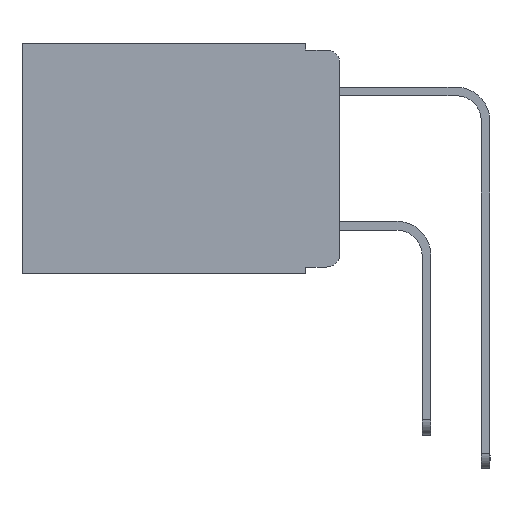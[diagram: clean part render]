
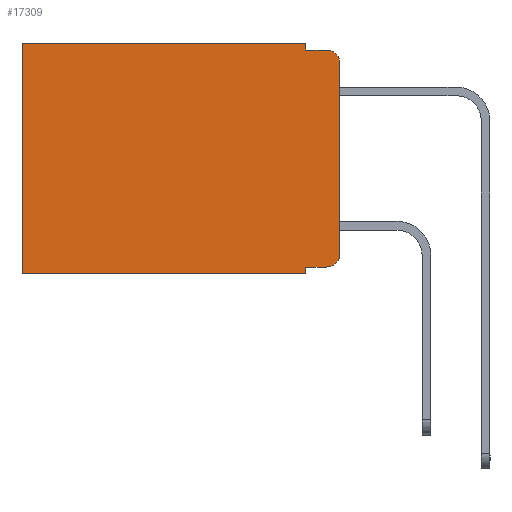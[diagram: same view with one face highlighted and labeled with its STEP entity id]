
A CAD part, left-side view. The second image highlights one B-rep face of the part: STEP entity #17309.
In plain terms, the highlighted planar face has unit normal (-1, 0, 0).
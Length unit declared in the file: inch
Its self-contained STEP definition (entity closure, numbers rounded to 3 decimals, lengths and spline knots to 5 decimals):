
#374 = VERTEX_POINT ( 'NONE', #19808 ) ;
#746 = AXIS2_PLACEMENT_3D ( 'NONE', #20291, #24024, #22146 ) ;
#793 = ORIENTED_EDGE ( 'NONE', *, *, #6416, .F. ) ;
#1081 = VERTEX_POINT ( 'NONE', #4981 ) ;
#1228 = CARTESIAN_POINT ( 'NONE',  ( 0.298, 0.473, -0.343 ) ) ;
#1316 = ORIENTED_EDGE ( 'NONE', *, *, #24752, .F. ) ;
#1496 = DIRECTION ( 'NONE',  ( 0., 0., -1. ) ) ;
#1647 = LINE ( 'NONE', #25582, #19690 ) ;
#1856 = CARTESIAN_POINT ( 'NONE',  ( 0.298, 0.051, -0.01 ) ) ;
#1897 = CARTESIAN_POINT ( 'NONE',  ( 0.298, 0., -0.313 ) ) ;
#3254 = DIRECTION ( 'NONE',  ( -1., 0., 0. ) ) ;
#3382 = DIRECTION ( 'NONE',  ( 0., 0., -1. ) ) ;
#3552 = LINE ( 'NONE', #17128, #19204 ) ;
#3572 = CARTESIAN_POINT ( 'NONE',  ( 0.298, 0., -0.343 ) ) ;
#3662 = FACE_OUTER_BOUND ( 'NONE', #3953, .T. ) ;
#3953 = EDGE_LOOP ( 'NONE', ( #14051, #13202, #793, #1316, #12378, #7994, #12371, #14739, #6467, #18732 ) ) ;
#4981 = CARTESIAN_POINT ( 'NONE',  ( 0.298, 0.051, 0. ) ) ;
#5083 = LINE ( 'NONE', #25435, #20933 ) ;
#5243 = VERTEX_POINT ( 'NONE', #13425 ) ;
#5363 = CIRCLE ( 'NONE', #21504, 0.02 ) ;
#6416 = EDGE_CURVE ( 'NONE', #20065, #8487, #1647, .T. ) ;
#6467 = ORIENTED_EDGE ( 'NONE', *, *, #23620, .T. ) ;
#6502 = EDGE_CURVE ( 'NONE', #1081, #5243, #12140, .T. ) ;
#6815 = VERTEX_POINT ( 'NONE', #1228 ) ;
#7169 = CARTESIAN_POINT ( 'NONE',  ( 0.298, 0.02, -0.01 ) ) ;
#7228 = DIRECTION ( 'NONE',  ( 0., -1., 0. ) ) ;
#7580 = EDGE_CURVE ( 'NONE', #374, #20787, #5363, .T. ) ;
#7651 = AXIS2_PLACEMENT_3D ( 'NONE', #17007, #13262, #10768 ) ;
#7803 = VECTOR ( 'NONE', #22971, 39.37008 ) ;
#7994 = ORIENTED_EDGE ( 'NONE', *, *, #25446, .T. ) ;
#8144 = EDGE_CURVE ( 'NONE', #11261, #20787, #21834, .T. ) ;
#8487 = VERTEX_POINT ( 'NONE', #7169 ) ;
#9439 = CARTESIAN_POINT ( 'NONE',  ( 0.298, 0.051, -0.343 ) ) ;
#9646 = CARTESIAN_POINT ( 'NONE',  ( 0.298, 0.02, -0.313 ) ) ;
#9894 = CARTESIAN_POINT ( 'NONE',  ( 0.298, 0., 0. ) ) ;
#9926 = VERTEX_POINT ( 'NONE', #9439 ) ;
#10768 = DIRECTION ( 'NONE',  ( 0., 0., -1. ) ) ;
#11077 = DIRECTION ( 'NONE',  ( 0., 0., -1. ) ) ;
#11261 = VERTEX_POINT ( 'NONE', #17435 ) ;
#12140 = LINE ( 'NONE', #9894, #23507 ) ;
#12351 = CARTESIAN_POINT ( 'NONE',  ( 0.298, 0.051, -0.333 ) ) ;
#12371 = ORIENTED_EDGE ( 'NONE', *, *, #14159, .F. ) ;
#12378 = ORIENTED_EDGE ( 'NONE', *, *, #6502, .T. ) ;
#12845 = CARTESIAN_POINT ( 'NONE',  ( 0.298, 0.473, 0. ) ) ;
#13202 = ORIENTED_EDGE ( 'NONE', *, *, #20263, .T. ) ;
#13262 = DIRECTION ( 'NONE',  ( -1., 0., 0. ) ) ;
#13425 = CARTESIAN_POINT ( 'NONE',  ( 0.298, 0.473, 0. ) ) ;
#13675 = DIRECTION ( 'NONE',  ( 0., 1., 0. ) ) ;
#14051 = ORIENTED_EDGE ( 'NONE', *, *, #8144, .F. ) ;
#14091 = DIRECTION ( 'NONE',  ( 0., -1., 0. ) ) ;
#14159 = EDGE_CURVE ( 'NONE', #9926, #6815, #21661, .T. ) ;
#14739 = ORIENTED_EDGE ( 'NONE', *, *, #23809, .F. ) ;
#15787 = VECTOR ( 'NONE', #14091, 39.37008 ) ;
#17007 = CARTESIAN_POINT ( 'NONE',  ( 0.298, 0.02, -0.03 ) ) ;
#17094 = LINE ( 'NONE', #12845, #7803 ) ;
#17128 = CARTESIAN_POINT ( 'NONE',  ( 0.298, 0.051, 0. ) ) ;
#17309 = ADVANCED_FACE ( 'NONE', ( #3662 ), #22421, .F. ) ;
#17435 = CARTESIAN_POINT ( 'NONE',  ( 0.298, 0., -0.03 ) ) ;
#18732 = ORIENTED_EDGE ( 'NONE', *, *, #7580, .T. ) ;
#19065 = CARTESIAN_POINT ( 'NONE',  ( 0.298, 0.051, -0.333 ) ) ;
#19204 = VECTOR ( 'NONE', #19257, 39.37008 ) ;
#19257 = DIRECTION ( 'NONE',  ( 0., 0., -1. ) ) ;
#19319 = VECTOR ( 'NONE', #1496, 39.37008 ) ;
#19453 = CARTESIAN_POINT ( 'NONE',  ( 0.298, 0., 0. ) ) ;
#19690 = VECTOR ( 'NONE', #7228, 39.37008 ) ;
#19808 = CARTESIAN_POINT ( 'NONE',  ( 0.298, 0.02, -0.333 ) ) ;
#20065 = VERTEX_POINT ( 'NONE', #1856 ) ;
#20078 = LINE ( 'NONE', #12351, #15787 ) ;
#20263 = EDGE_CURVE ( 'NONE', #11261, #8487, #20398, .T. ) ;
#20291 = CARTESIAN_POINT ( 'NONE',  ( 0.298, 0., 0. ) ) ;
#20398 = CIRCLE ( 'NONE', #7651, 0.02 ) ;
#20787 = VERTEX_POINT ( 'NONE', #1897 ) ;
#20933 = VECTOR ( 'NONE', #11077, 39.37008 ) ;
#21504 = AXIS2_PLACEMENT_3D ( 'NONE', #9646, #3254, #3382 ) ;
#21661 = LINE ( 'NONE', #3572, #26151 ) ;
#21834 = LINE ( 'NONE', #19453, #19319 ) ;
#22146 = DIRECTION ( 'NONE',  ( 0., 0., -1. ) ) ;
#22421 = PLANE ( 'NONE',  #746 ) ;
#22971 = DIRECTION ( 'NONE',  ( 0., 0., -1. ) ) ;
#23507 = VECTOR ( 'NONE', #24525, 39.37008 ) ;
#23620 = EDGE_CURVE ( 'NONE', #26083, #374, #20078, .T. ) ;
#23809 = EDGE_CURVE ( 'NONE', #26083, #9926, #3552, .T. ) ;
#24024 = DIRECTION ( 'NONE',  ( 1., 0., 0. ) ) ;
#24525 = DIRECTION ( 'NONE',  ( 0., 1., 0. ) ) ;
#24752 = EDGE_CURVE ( 'NONE', #1081, #20065, #5083, .T. ) ;
#25435 = CARTESIAN_POINT ( 'NONE',  ( 0.298, 0.051, 0. ) ) ;
#25446 = EDGE_CURVE ( 'NONE', #5243, #6815, #17094, .T. ) ;
#25582 = CARTESIAN_POINT ( 'NONE',  ( 0.298, 0.051, -0.01 ) ) ;
#26083 = VERTEX_POINT ( 'NONE', #19065 ) ;
#26151 = VECTOR ( 'NONE', #13675, 39.37008 ) ;
